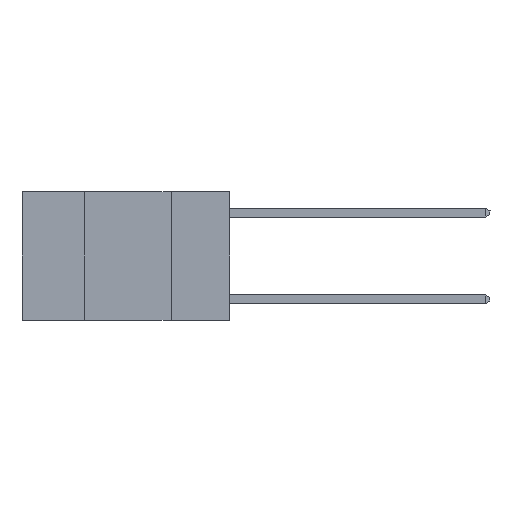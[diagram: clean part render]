
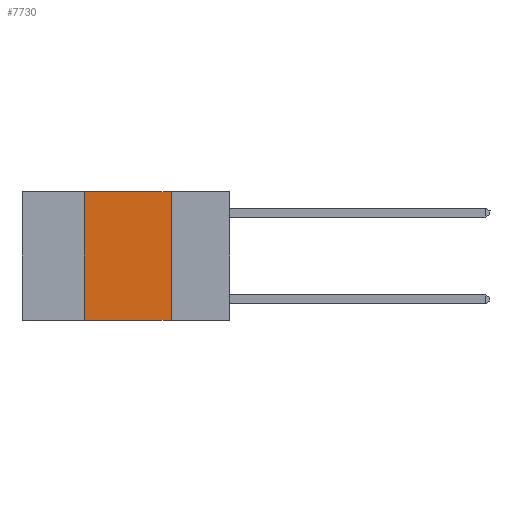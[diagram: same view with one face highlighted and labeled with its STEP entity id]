
A CAD part, left-side view. The second image highlights one B-rep face of the part: STEP entity #7730.
In plain terms, the highlighted planar face has unit normal (-1, 0, 0).
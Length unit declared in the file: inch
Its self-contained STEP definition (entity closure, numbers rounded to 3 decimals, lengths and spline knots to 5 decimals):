
#41 = ORIENTED_EDGE ( 'NONE', *, *, #16277, .F. ) ;
#340 = DIRECTION ( 'NONE',  ( 1., 0., 0. ) ) ;
#747 = DIRECTION ( 'NONE',  ( 0., 0., -1. ) ) ;
#1188 = AXIS2_PLACEMENT_3D ( 'NONE', #7787, #340, #11997 ) ;
#1890 = ORIENTED_EDGE ( 'NONE', *, *, #10016, .F. ) ;
#2444 = CARTESIAN_POINT ( 'NONE',  ( 0., 0.42, -0.37 ) ) ;
#2508 = VERTEX_POINT ( 'NONE', #14607 ) ;
#3732 = EDGE_LOOP ( 'NONE', ( #1890, #41, #9177, #5252 ) ) ;
#4032 = VERTEX_POINT ( 'NONE', #2444 ) ;
#5252 = ORIENTED_EDGE ( 'NONE', *, *, #18492, .T. ) ;
#7084 = VERTEX_POINT ( 'NONE', #16394 ) ;
#7730 = ADVANCED_FACE ( 'NONE', ( #13486 ), #8956, .F. ) ;
#7787 = CARTESIAN_POINT ( 'NONE',  ( 0., 0.6, 0. ) ) ;
#7844 = CARTESIAN_POINT ( 'NONE',  ( 0., 0.6, 0. ) ) ;
#8044 = DIRECTION ( 'NONE',  ( 0., -1., 0. ) ) ;
#8281 = LINE ( 'NONE', #9663, #9289 ) ;
#8478 = EDGE_CURVE ( 'NONE', #4032, #2508, #17977, .T. ) ;
#8698 = VERTEX_POINT ( 'NONE', #18946 ) ;
#8956 = PLANE ( 'NONE',  #1188 ) ;
#9177 = ORIENTED_EDGE ( 'NONE', *, *, #8478, .F. ) ;
#9289 = VECTOR ( 'NONE', #747, 39.37008 ) ;
#9663 = CARTESIAN_POINT ( 'NONE',  ( 0., 0.17, 0. ) ) ;
#10016 = EDGE_CURVE ( 'NONE', #7084, #8698, #8281, .T. ) ;
#10838 = CARTESIAN_POINT ( 'NONE',  ( 0., 0.6, -0.37 ) ) ;
#11997 = DIRECTION ( 'NONE',  ( 0., 0., -1. ) ) ;
#12121 = LINE ( 'NONE', #10838, #16418 ) ;
#12317 = DIRECTION ( 'NONE',  ( 0., -1., 0. ) ) ;
#12370 = VECTOR ( 'NONE', #18076, 39.37008 ) ;
#12498 = VECTOR ( 'NONE', #8044, 39.37008 ) ;
#13120 = CARTESIAN_POINT ( 'NONE',  ( 0., 0.42, 0. ) ) ;
#13486 = FACE_OUTER_BOUND ( 'NONE', #3732, .T. ) ;
#14607 = CARTESIAN_POINT ( 'NONE',  ( 0., 0.42, 0. ) ) ;
#16277 = EDGE_CURVE ( 'NONE', #2508, #7084, #16816, .T. ) ;
#16394 = CARTESIAN_POINT ( 'NONE',  ( 0., 0.17, 0. ) ) ;
#16418 = VECTOR ( 'NONE', #12317, 39.37008 ) ;
#16816 = LINE ( 'NONE', #7844, #12498 ) ;
#17977 = LINE ( 'NONE', #13120, #12370 ) ;
#18076 = DIRECTION ( 'NONE',  ( 0., 0., 1. ) ) ;
#18492 = EDGE_CURVE ( 'NONE', #4032, #8698, #12121, .T. ) ;
#18946 = CARTESIAN_POINT ( 'NONE',  ( 0., 0.17, -0.37 ) ) ;
